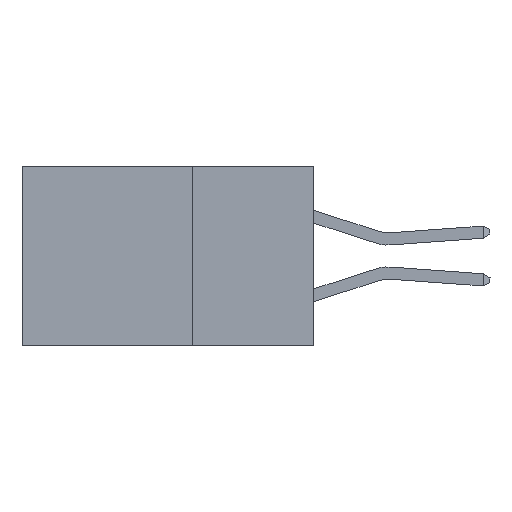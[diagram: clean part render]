
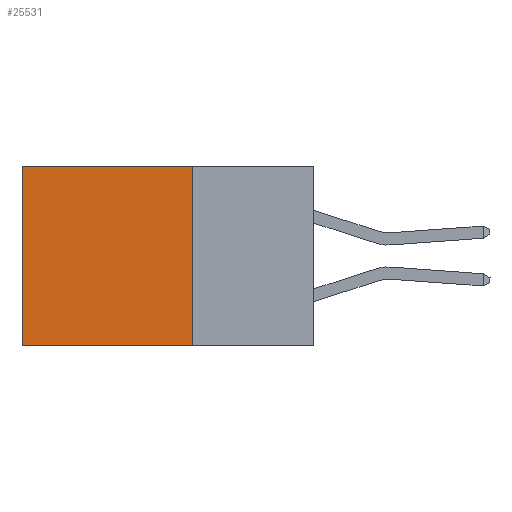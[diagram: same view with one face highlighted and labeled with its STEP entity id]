
A CAD part, left-side view. The second image highlights one B-rep face of the part: STEP entity #25531.
In plain terms, the highlighted planar face has unit normal (-1, 0, 0).
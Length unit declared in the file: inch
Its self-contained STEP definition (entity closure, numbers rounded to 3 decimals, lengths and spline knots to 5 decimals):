
#1303 = CARTESIAN_POINT ( 'NONE',  ( 0.2875, 0.6, 0. ) ) ;
#1778 = ORIENTED_EDGE ( 'NONE', *, *, #9900, .F. ) ;
#2038 = VECTOR ( 'NONE', #29132, 39.37008 ) ;
#2707 = CARTESIAN_POINT ( 'NONE',  ( 0.2875, 0.25, 0. ) ) ;
#3416 = CARTESIAN_POINT ( 'NONE',  ( 0.2875, 0.6, 0. ) ) ;
#4900 = LINE ( 'NONE', #16264, #15522 ) ;
#5620 = AXIS2_PLACEMENT_3D ( 'NONE', #22924, #17176, #28681 ) ;
#7494 = CARTESIAN_POINT ( 'NONE',  ( 0.2875, 0.6, -0.37 ) ) ;
#8578 = PLANE ( 'NONE',  #5620 ) ;
#8595 = VERTEX_POINT ( 'NONE', #7494 ) ;
#9900 = EDGE_CURVE ( 'NONE', #28986, #8595, #4900, .T. ) ;
#11204 = FACE_OUTER_BOUND ( 'NONE', #28351, .T. ) ;
#11463 = EDGE_CURVE ( 'NONE', #11925, #16915, #13738, .T. ) ;
#11925 = VERTEX_POINT ( 'NONE', #2707 ) ;
#13738 = LINE ( 'NONE', #30866, #25647 ) ;
#15448 = EDGE_CURVE ( 'NONE', #11925, #28986, #34718, .T. ) ;
#15522 = VECTOR ( 'NONE', #27970, 39.37008 ) ;
#16264 = CARTESIAN_POINT ( 'NONE',  ( 0.2875, 0.25, -0.37 ) ) ;
#16915 = VERTEX_POINT ( 'NONE', #3416 ) ;
#17095 = DIRECTION ( 'NONE',  ( 0., 1., 0. ) ) ;
#17176 = DIRECTION ( 'NONE',  ( 1., 0., 0. ) ) ;
#17793 = CARTESIAN_POINT ( 'NONE',  ( 0.2875, 0.25, 0. ) ) ;
#19209 = ORIENTED_EDGE ( 'NONE', *, *, #11463, .T. ) ;
#21204 = CARTESIAN_POINT ( 'NONE',  ( 0.2875, 0.25, -0.37 ) ) ;
#21926 = DIRECTION ( 'NONE',  ( 0., 0., -1. ) ) ;
#22924 = CARTESIAN_POINT ( 'NONE',  ( 0.2875, 0.25, 0. ) ) ;
#24747 = VECTOR ( 'NONE', #21926, 39.37008 ) ;
#25531 = ADVANCED_FACE ( 'NONE', ( #11204 ), #8578, .F. ) ;
#25647 = VECTOR ( 'NONE', #17095, 39.37008 ) ;
#27616 = EDGE_CURVE ( 'NONE', #16915, #8595, #33284, .T. ) ;
#27970 = DIRECTION ( 'NONE',  ( 0., 1., 0. ) ) ;
#28351 = EDGE_LOOP ( 'NONE', ( #29307, #1778, #30968, #19209 ) ) ;
#28681 = DIRECTION ( 'NONE',  ( 0., 0., -1. ) ) ;
#28986 = VERTEX_POINT ( 'NONE', #21204 ) ;
#29132 = DIRECTION ( 'NONE',  ( 0., 0., -1. ) ) ;
#29307 = ORIENTED_EDGE ( 'NONE', *, *, #27616, .T. ) ;
#30866 = CARTESIAN_POINT ( 'NONE',  ( 0.2875, 0.25, 0. ) ) ;
#30968 = ORIENTED_EDGE ( 'NONE', *, *, #15448, .F. ) ;
#33284 = LINE ( 'NONE', #1303, #24747 ) ;
#34718 = LINE ( 'NONE', #17793, #2038 ) ;
